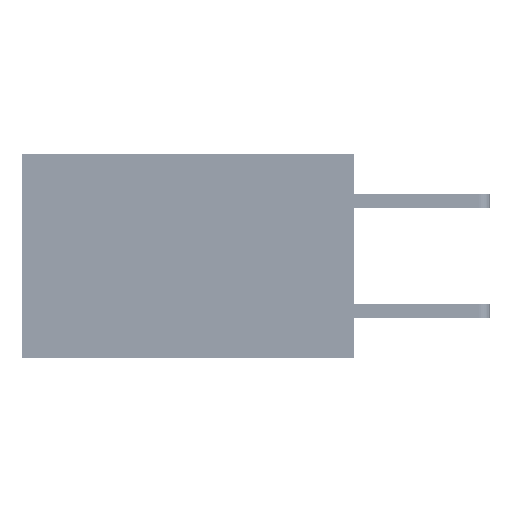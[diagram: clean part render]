
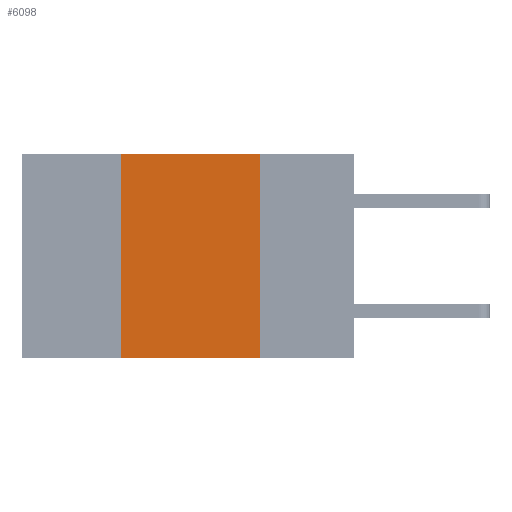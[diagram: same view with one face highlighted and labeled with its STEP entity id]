
A CAD part, left-side view. The second image highlights one B-rep face of the part: STEP entity #6098.
In plain terms, the highlighted planar face has unit normal (-1, 0, 0).
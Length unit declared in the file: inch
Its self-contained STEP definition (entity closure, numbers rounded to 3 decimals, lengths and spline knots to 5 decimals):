
#306 = VERTEX_POINT ( 'NONE', #33091 ) ;
#392 = LINE ( 'NONE', #29276, #12187 ) ;
#838 = DIRECTION ( 'NONE',  ( 0., 0., -1. ) ) ;
#1213 = VERTEX_POINT ( 'NONE', #11596 ) ;
#1372 = ORIENTED_EDGE ( 'NONE', *, *, #29719, .T. ) ;
#2858 = EDGE_CURVE ( 'NONE', #306, #1213, #392, .T. ) ;
#2954 = VECTOR ( 'NONE', #39487, 39.37008 ) ;
#4183 = AXIS2_PLACEMENT_3D ( 'NONE', #4497, #10757, #838 ) ;
#4497 = CARTESIAN_POINT ( 'NONE',  ( 0., 0.6, 0. ) ) ;
#6098 = ADVANCED_FACE ( 'NONE', ( #17402 ), #36834, .F. ) ;
#7403 = ORIENTED_EDGE ( 'NONE', *, *, #2858, .F. ) ;
#9654 = DIRECTION ( 'NONE',  ( 0., 0., -1. ) ) ;
#10757 = DIRECTION ( 'NONE',  ( 1., 0., 0. ) ) ;
#11240 = VECTOR ( 'NONE', #30039, 39.37008 ) ;
#11596 = CARTESIAN_POINT ( 'NONE',  ( 0., 0.17, -0.37 ) ) ;
#12187 = VECTOR ( 'NONE', #9654, 39.37008 ) ;
#13621 = CARTESIAN_POINT ( 'NONE',  ( 0., 0.6, 0. ) ) ;
#14489 = CARTESIAN_POINT ( 'NONE',  ( 0., 0.42, 0. ) ) ;
#17402 = FACE_OUTER_BOUND ( 'NONE', #21692, .T. ) ;
#19433 = CARTESIAN_POINT ( 'NONE',  ( 0., 0.42, 0. ) ) ;
#19570 = VERTEX_POINT ( 'NONE', #22070 ) ;
#21527 = ORIENTED_EDGE ( 'NONE', *, *, #22821, .F. ) ;
#21692 = EDGE_LOOP ( 'NONE', ( #7403, #24248, #21527, #1372 ) ) ;
#22005 = LINE ( 'NONE', #41003, #30240 ) ;
#22070 = CARTESIAN_POINT ( 'NONE',  ( 0., 0.42, -0.37 ) ) ;
#22821 = EDGE_CURVE ( 'NONE', #19570, #38731, #40144, .T. ) ;
#24248 = ORIENTED_EDGE ( 'NONE', *, *, #35798, .F. ) ;
#29276 = CARTESIAN_POINT ( 'NONE',  ( 0., 0.17, 0. ) ) ;
#29719 = EDGE_CURVE ( 'NONE', #19570, #1213, #22005, .T. ) ;
#30039 = DIRECTION ( 'NONE',  ( 0., 0., 1. ) ) ;
#30240 = VECTOR ( 'NONE', #37776, 39.37008 ) ;
#30442 = LINE ( 'NONE', #13621, #2954 ) ;
#33091 = CARTESIAN_POINT ( 'NONE',  ( 0., 0.17, 0. ) ) ;
#35798 = EDGE_CURVE ( 'NONE', #38731, #306, #30442, .T. ) ;
#36834 = PLANE ( 'NONE',  #4183 ) ;
#37776 = DIRECTION ( 'NONE',  ( 0., -1., 0. ) ) ;
#38731 = VERTEX_POINT ( 'NONE', #19433 ) ;
#39487 = DIRECTION ( 'NONE',  ( 0., -1., 0. ) ) ;
#40144 = LINE ( 'NONE', #14489, #11240 ) ;
#41003 = CARTESIAN_POINT ( 'NONE',  ( 0., 0.6, -0.37 ) ) ;
